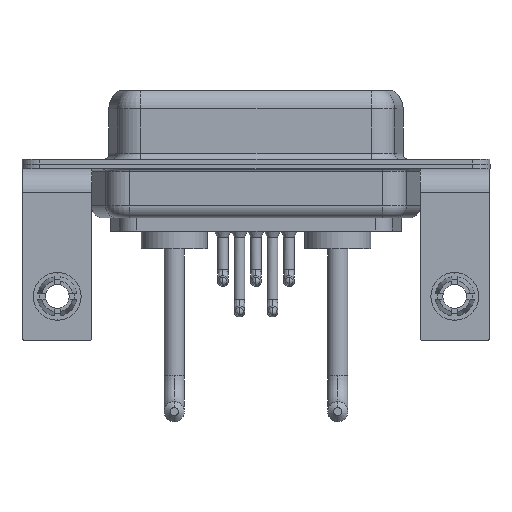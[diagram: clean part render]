
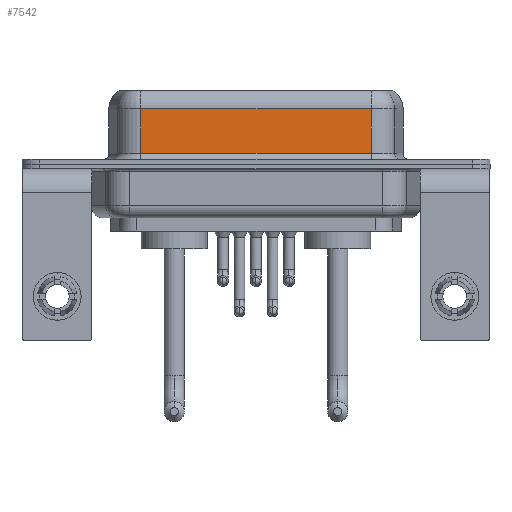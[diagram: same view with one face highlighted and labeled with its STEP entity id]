
A CAD part, front view. The second image highlights one B-rep face of the part: STEP entity #7542.
In plain terms, the highlighted planar face has unit normal (0, -1, 0).
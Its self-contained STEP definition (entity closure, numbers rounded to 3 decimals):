
#125 = DIRECTION ( 'NONE',  ( 0., 0., -1. ) ) ;
#767 = LINE ( 'NONE', #9835, #10594 ) ;
#903 = DIRECTION ( 'NONE',  ( -1., 0., 0. ) ) ;
#1459 = PLANE ( 'NONE',  #18666 ) ;
#1545 = VERTEX_POINT ( 'NONE', #8193 ) ;
#1813 = ORIENTED_EDGE ( 'NONE', *, *, #16531, .T. ) ;
#2651 = ORIENTED_EDGE ( 'NONE', *, *, #11864, .F. ) ;
#3265 = VECTOR ( 'NONE', #17733, 1000. ) ;
#3577 = VECTOR ( 'NONE', #903, 1000. ) ;
#4194 = LINE ( 'NONE', #11878, #3265 ) ;
#4849 = VERTEX_POINT ( 'NONE', #14115 ) ;
#4956 = CARTESIAN_POINT ( 'NONE',  ( 7.013, -3.95, 0.9 ) ) ;
#5164 = ORIENTED_EDGE ( 'NONE', *, *, #15991, .T. ) ;
#5848 = CARTESIAN_POINT ( 'NONE',  ( 26.287, -3.95, 6.4 ) ) ;
#5993 = LINE ( 'NONE', #11917, #7040 ) ;
#7026 = DIRECTION ( 'NONE',  ( 0., 0., -1. ) ) ;
#7040 = VECTOR ( 'NONE', #125, 1000. ) ;
#7542 = ADVANCED_FACE ( 'NONE', ( #19086 ), #1459, .F. ) ;
#8193 = CARTESIAN_POINT ( 'NONE',  ( 26.287, -3.95, 4.65 ) ) ;
#8325 = CARTESIAN_POINT ( 'NONE',  ( 26.287, -3.95, 4.65 ) ) ;
#8869 = DIRECTION ( 'NONE',  ( 0., 1., 0. ) ) ;
#9775 = LINE ( 'NONE', #8325, #3577 ) ;
#9835 = CARTESIAN_POINT ( 'NONE',  ( 26.287, -3.95, 6.4 ) ) ;
#10549 = EDGE_LOOP ( 'NONE', ( #2651, #5164, #18158, #1813 ) ) ;
#10594 = VECTOR ( 'NONE', #7026, 1000. ) ;
#11352 = EDGE_CURVE ( 'NONE', #13609, #19044, #5993, .T. ) ;
#11864 = EDGE_CURVE ( 'NONE', #1545, #4849, #767, .T. ) ;
#11878 = CARTESIAN_POINT ( 'NONE',  ( 26.287, -3.95, 0.9 ) ) ;
#11917 = CARTESIAN_POINT ( 'NONE',  ( 7.013, -3.95, 6.4 ) ) ;
#13609 = VERTEX_POINT ( 'NONE', #18586 ) ;
#14115 = CARTESIAN_POINT ( 'NONE',  ( 26.287, -3.95, 0.9 ) ) ;
#15991 = EDGE_CURVE ( 'NONE', #1545, #13609, #9775, .T. ) ;
#16370 = DIRECTION ( 'NONE',  ( 0., 0., 1. ) ) ;
#16531 = EDGE_CURVE ( 'NONE', #19044, #4849, #4194, .T. ) ;
#17733 = DIRECTION ( 'NONE',  ( 1., 0., 0. ) ) ;
#18158 = ORIENTED_EDGE ( 'NONE', *, *, #11352, .T. ) ;
#18586 = CARTESIAN_POINT ( 'NONE',  ( 7.013, -3.95, 4.65 ) ) ;
#18666 = AXIS2_PLACEMENT_3D ( 'NONE', #5848, #8869, #16370 ) ;
#19044 = VERTEX_POINT ( 'NONE', #4956 ) ;
#19086 = FACE_OUTER_BOUND ( 'NONE', #10549, .T. ) ;
